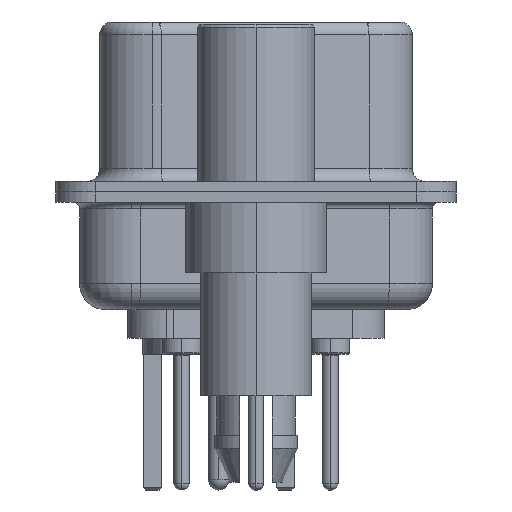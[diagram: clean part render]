
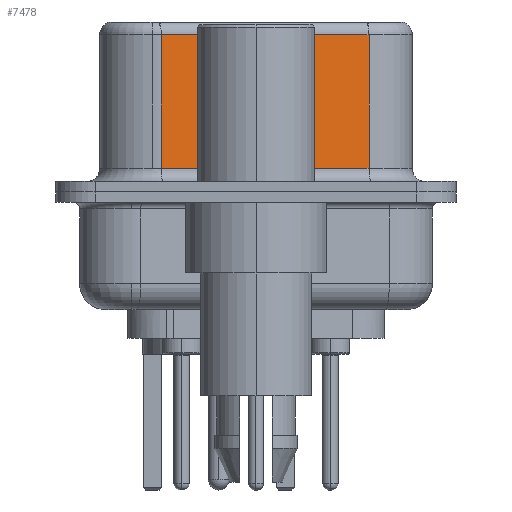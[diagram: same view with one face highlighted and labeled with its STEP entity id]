
A CAD part, left-side view. The second image highlights one B-rep face of the part: STEP entity #7478.
In plain terms, the highlighted planar face has unit normal (-0.985, -0.174, 0).
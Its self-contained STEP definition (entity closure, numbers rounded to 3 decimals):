
#61 = VECTOR ( 'NONE', #23239, 1000. ) ;
#972 = CARTESIAN_POINT ( 'NONE',  ( 5.132, -4.322, 6.52 ) ) ;
#1313 = CARTESIAN_POINT ( 'NONE',  ( 5.132, -4.322, 0.9 ) ) ;
#2785 = CARTESIAN_POINT ( 'NONE',  ( 3.73, 3.628, 0.9 ) ) ;
#3314 = VERTEX_POINT ( 'NONE', #2785 ) ;
#4329 = DIRECTION ( 'NONE',  ( 0.174, -0.985, 0. ) ) ;
#4876 = LINE ( 'NONE', #9398, #6047 ) ;
#6047 = VECTOR ( 'NONE', #22081, 1000. ) ;
#6768 = VECTOR ( 'NONE', #15186, 1000. ) ;
#7467 = FACE_OUTER_BOUND ( 'NONE', #19656, .T. ) ;
#7478 = ADVANCED_FACE ( 'NONE', ( #7467 ), #24914, .F. ) ;
#9398 = CARTESIAN_POINT ( 'NONE',  ( 3.73, 3.628, 6.52 ) ) ;
#9402 = CARTESIAN_POINT ( 'NONE',  ( 5.132, -4.322, 0.9 ) ) ;
#9615 = ORIENTED_EDGE ( 'NONE', *, *, #20358, .T. ) ;
#11920 = EDGE_CURVE ( 'NONE', #19010, #25376, #21650, .T. ) ;
#12991 = LINE ( 'NONE', #27830, #6768 ) ;
#13153 = VERTEX_POINT ( 'NONE', #23570 ) ;
#14754 = CARTESIAN_POINT ( 'NONE',  ( 5.132, -4.322, 6.52 ) ) ;
#15186 = DIRECTION ( 'NONE',  ( -0.174, 0.985, 0. ) ) ;
#16122 = AXIS2_PLACEMENT_3D ( 'NONE', #14754, #17168, #25022 ) ;
#16964 = VECTOR ( 'NONE', #4329, 1000. ) ;
#17168 = DIRECTION ( 'NONE',  ( 0.985, 0.174, 0. ) ) ;
#19010 = VERTEX_POINT ( 'NONE', #25027 ) ;
#19656 = EDGE_LOOP ( 'NONE', ( #31173, #27913, #9615, #29623 ) ) ;
#20358 = EDGE_CURVE ( 'NONE', #13153, #3314, #4876, .T. ) ;
#21650 = LINE ( 'NONE', #972, #61 ) ;
#22081 = DIRECTION ( 'NONE',  ( 0., 0., -1. ) ) ;
#23239 = DIRECTION ( 'NONE',  ( 0., 0., -1. ) ) ;
#23570 = CARTESIAN_POINT ( 'NONE',  ( 3.73, 3.628, 6.02 ) ) ;
#23670 = EDGE_CURVE ( 'NONE', #3314, #25376, #23989, .T. ) ;
#23911 = EDGE_CURVE ( 'NONE', #19010, #13153, #12991, .T. ) ;
#23989 = LINE ( 'NONE', #9402, #16964 ) ;
#24914 = PLANE ( 'NONE',  #16122 ) ;
#25022 = DIRECTION ( 'NONE',  ( -0.174, 0.985, 0. ) ) ;
#25027 = CARTESIAN_POINT ( 'NONE',  ( 5.132, -4.322, 6.02 ) ) ;
#25376 = VERTEX_POINT ( 'NONE', #1313 ) ;
#27830 = CARTESIAN_POINT ( 'NONE',  ( 5.132, -4.322, 6.02 ) ) ;
#27913 = ORIENTED_EDGE ( 'NONE', *, *, #23911, .T. ) ;
#29623 = ORIENTED_EDGE ( 'NONE', *, *, #23670, .T. ) ;
#31173 = ORIENTED_EDGE ( 'NONE', *, *, #11920, .F. ) ;
